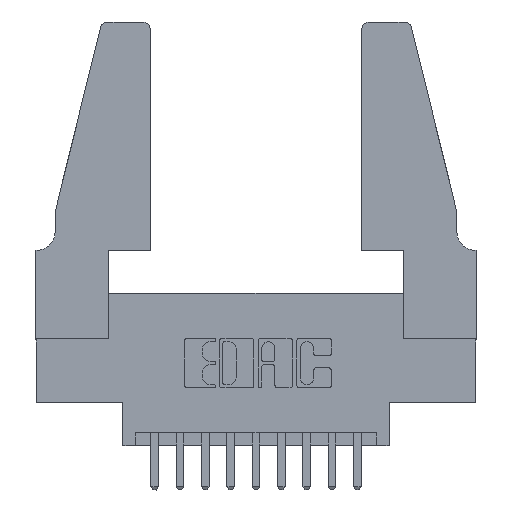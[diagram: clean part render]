
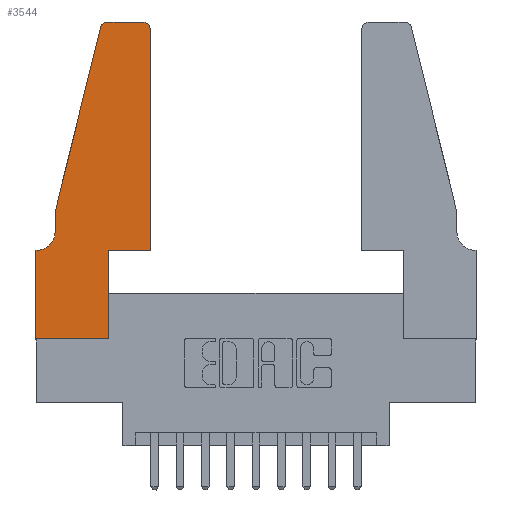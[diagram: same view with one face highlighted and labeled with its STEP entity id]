
A CAD part, top view. The second image highlights one B-rep face of the part: STEP entity #3544.
In plain terms, the highlighted planar face has unit normal (0, 0, 1).
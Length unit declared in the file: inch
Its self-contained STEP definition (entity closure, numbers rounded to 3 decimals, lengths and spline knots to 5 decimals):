
#11 = PLANE ( 'NONE',  #11971 ) ;
#271 = VERTEX_POINT ( 'NONE', #8611 ) ;
#347 = DIRECTION ( 'NONE',  ( 0., 0., 1. ) ) ;
#724 = CIRCLE ( 'NONE', #10627, 0.03 ) ;
#832 = ORIENTED_EDGE ( 'NONE', *, *, #2990, .T. ) ;
#902 = DIRECTION ( 'NONE',  ( 1., 0., 0. ) ) ;
#943 = EDGE_LOOP ( 'NONE', ( #10117, #832, #9322, #13152, #11393, #12321, #13393, #6282, #8156, #2791, #6903, #8405 ) ) ;
#1038 = CARTESIAN_POINT ( 'NONE',  ( 0.0755, 0.5, 0.37 ) ) ;
#1140 = DIRECTION ( 'NONE',  ( 1., 0., 0. ) ) ;
#1196 = VECTOR ( 'NONE', #4910, 39.37008 ) ;
#1254 = VECTOR ( 'NONE', #7348, 39.37008 ) ;
#1338 = CARTESIAN_POINT ( 'NONE',  ( 0.0755, 0.42, 0.37 ) ) ;
#1480 = VERTEX_POINT ( 'NONE', #10577 ) ;
#1506 = LINE ( 'NONE', #2117, #10933 ) ;
#1592 = VERTEX_POINT ( 'NONE', #1338 ) ;
#1660 = CARTESIAN_POINT ( 'NONE',  ( 0.284, 1.22, 0.37 ) ) ;
#1732 = LINE ( 'NONE', #3365, #9635 ) ;
#2000 = VECTOR ( 'NONE', #11751, 39.37008 ) ;
#2117 = CARTESIAN_POINT ( 'NONE',  ( 0., 0., 0.37 ) ) ;
#2146 = CARTESIAN_POINT ( 'NONE',  ( 0.0055, 0.42, 0.37 ) ) ;
#2154 = EDGE_CURVE ( 'NONE', #7648, #9008, #4649, .T. ) ;
#2463 = CARTESIAN_POINT ( 'NONE',  ( 0., 0., 0.37 ) ) ;
#2723 = LINE ( 'NONE', #11397, #1196 ) ;
#2791 = ORIENTED_EDGE ( 'NONE', *, *, #5411, .T. ) ;
#2903 = CARTESIAN_POINT ( 'NONE',  ( 0.0755, 0.5, 0.37 ) ) ;
#2966 = DIRECTION ( 'NONE',  ( 1., 0., 0. ) ) ;
#2990 = EDGE_CURVE ( 'NONE', #10329, #11766, #10034, .T. ) ;
#3365 = CARTESIAN_POINT ( 'NONE',  ( 0.4505, 0.35, 0.37 ) ) ;
#3455 = LINE ( 'NONE', #1038, #1254 ) ;
#3518 = EDGE_CURVE ( 'NONE', #11766, #9874, #3455, .T. ) ;
#3544 = ADVANCED_FACE ( 'NONE', ( #12017 ), #11, .T. ) ;
#3600 = CIRCLE ( 'NONE', #7762, 0.07 ) ;
#3763 = VERTEX_POINT ( 'NONE', #7922 ) ;
#4108 = CARTESIAN_POINT ( 'NONE',  ( 0.0755, 0.35, 0.37 ) ) ;
#4649 = LINE ( 'NONE', #6058, #6681 ) ;
#4788 = EDGE_CURVE ( 'NONE', #3763, #13120, #13352, .T. ) ;
#4804 = VECTOR ( 'NONE', #7295, 39.37008 ) ;
#4910 = DIRECTION ( 'NONE',  ( -1., 0., 0. ) ) ;
#4913 = VERTEX_POINT ( 'NONE', #5418 ) ;
#4914 = EDGE_CURVE ( 'NONE', #1592, #4913, #3600, .T. ) ;
#5411 = EDGE_CURVE ( 'NONE', #13120, #7648, #1732, .T. ) ;
#5418 = CARTESIAN_POINT ( 'NONE',  ( 0.0055, 0.35, 0.37 ) ) ;
#5570 = CARTESIAN_POINT ( 'NONE',  ( 0.4505, 1.22, 0.37 ) ) ;
#6058 = CARTESIAN_POINT ( 'NONE',  ( 0.4505, 0.35, 0.37 ) ) ;
#6277 = DIRECTION ( 'NONE',  ( 0., 1., 0. ) ) ;
#6282 = ORIENTED_EDGE ( 'NONE', *, *, #13357, .T. ) ;
#6681 = VECTOR ( 'NONE', #6955, 39.37008 ) ;
#6903 = ORIENTED_EDGE ( 'NONE', *, *, #2154, .T. ) ;
#6913 = VECTOR ( 'NONE', #12716, 39.37008 ) ;
#6955 = DIRECTION ( 'NONE',  ( 0., 1., 0. ) ) ;
#6969 = VERTEX_POINT ( 'NONE', #8682 ) ;
#7295 = DIRECTION ( 'NONE',  ( 0., -1., 0. ) ) ;
#7348 = DIRECTION ( 'NONE',  ( -0.239, -0.971, 0. ) ) ;
#7551 = LINE ( 'NONE', #2463, #2000 ) ;
#7648 = VERTEX_POINT ( 'NONE', #9085 ) ;
#7762 = AXIS2_PLACEMENT_3D ( 'NONE', #2146, #8698, #11816 ) ;
#7816 = CARTESIAN_POINT ( 'NONE',  ( 0.4205, 1.22, 0.37 ) ) ;
#7920 = DIRECTION ( 'NONE',  ( 0., 0., 1. ) ) ;
#7922 = CARTESIAN_POINT ( 'NONE',  ( 0.2865, 0., 0.37 ) ) ;
#8156 = ORIENTED_EDGE ( 'NONE', *, *, #4788, .T. ) ;
#8405 = ORIENTED_EDGE ( 'NONE', *, *, #11400, .T. ) ;
#8611 = CARTESIAN_POINT ( 'NONE',  ( 0., 0., 0.37 ) ) ;
#8682 = CARTESIAN_POINT ( 'NONE',  ( 0., 0.35, 0.37 ) ) ;
#8698 = DIRECTION ( 'NONE',  ( 0., 0., -1. ) ) ;
#8791 = CARTESIAN_POINT ( 'NONE',  ( 0.25487, 1.22718, 0.37 ) ) ;
#8827 = EDGE_CURVE ( 'NONE', #9874, #1592, #10031, .T. ) ;
#9008 = VERTEX_POINT ( 'NONE', #5570 ) ;
#9085 = CARTESIAN_POINT ( 'NONE',  ( 0.4505, 0.35, 0.37 ) ) ;
#9322 = ORIENTED_EDGE ( 'NONE', *, *, #3518, .T. ) ;
#9427 = CARTESIAN_POINT ( 'NONE',  ( 0.2865, 0.35, 0.37 ) ) ;
#9502 = DIRECTION ( 'NONE',  ( 0., -1., 0. ) ) ;
#9596 = CARTESIAN_POINT ( 'NONE',  ( 0., 0.35, 0.37 ) ) ;
#9635 = VECTOR ( 'NONE', #1140, 39.37008 ) ;
#9645 = DIRECTION ( 'NONE',  ( 0., 0., 1. ) ) ;
#9874 = VERTEX_POINT ( 'NONE', #11444 ) ;
#10031 = LINE ( 'NONE', #2903, #4804 ) ;
#10034 = CIRCLE ( 'NONE', #11336, 0.03 ) ;
#10117 = ORIENTED_EDGE ( 'NONE', *, *, #12135, .T. ) ;
#10329 = VERTEX_POINT ( 'NONE', #10596 ) ;
#10357 = VECTOR ( 'NONE', #6277, 39.37008 ) ;
#10577 = CARTESIAN_POINT ( 'NONE',  ( 0.4205, 1.25, 0.37 ) ) ;
#10596 = CARTESIAN_POINT ( 'NONE',  ( 0.284, 1.25, 0.37 ) ) ;
#10627 = AXIS2_PLACEMENT_3D ( 'NONE', #7816, #347, #13266 ) ;
#10933 = VECTOR ( 'NONE', #9502, 39.37008 ) ;
#11279 = LINE ( 'NONE', #4108, #6913 ) ;
#11336 = AXIS2_PLACEMENT_3D ( 'NONE', #1660, #7920, #2966 ) ;
#11393 = ORIENTED_EDGE ( 'NONE', *, *, #4914, .T. ) ;
#11397 = CARTESIAN_POINT ( 'NONE',  ( 0.2605, 1.25, 0.37 ) ) ;
#11400 = EDGE_CURVE ( 'NONE', #9008, #1480, #724, .T. ) ;
#11444 = CARTESIAN_POINT ( 'NONE',  ( 0.0755, 0.5, 0.37 ) ) ;
#11634 = CARTESIAN_POINT ( 'NONE',  ( 0.2865, 0.35, 0.37 ) ) ;
#11751 = DIRECTION ( 'NONE',  ( 1., 0., 0. ) ) ;
#11766 = VERTEX_POINT ( 'NONE', #8791 ) ;
#11816 = DIRECTION ( 'NONE',  ( -1., 0., 0. ) ) ;
#11971 = AXIS2_PLACEMENT_3D ( 'NONE', #9596, #9645, #902 ) ;
#12017 = FACE_OUTER_BOUND ( 'NONE', #943, .T. ) ;
#12135 = EDGE_CURVE ( 'NONE', #1480, #10329, #2723, .T. ) ;
#12173 = EDGE_CURVE ( 'NONE', #4913, #6969, #11279, .T. ) ;
#12321 = ORIENTED_EDGE ( 'NONE', *, *, #12173, .T. ) ;
#12716 = DIRECTION ( 'NONE',  ( -1., 0., 0. ) ) ;
#13120 = VERTEX_POINT ( 'NONE', #9427 ) ;
#13152 = ORIENTED_EDGE ( 'NONE', *, *, #8827, .T. ) ;
#13180 = EDGE_CURVE ( 'NONE', #6969, #271, #1506, .T. ) ;
#13266 = DIRECTION ( 'NONE',  ( 1., 0., 0. ) ) ;
#13352 = LINE ( 'NONE', #11634, #10357 ) ;
#13357 = EDGE_CURVE ( 'NONE', #271, #3763, #7551, .T. ) ;
#13393 = ORIENTED_EDGE ( 'NONE', *, *, #13180, .T. ) ;
